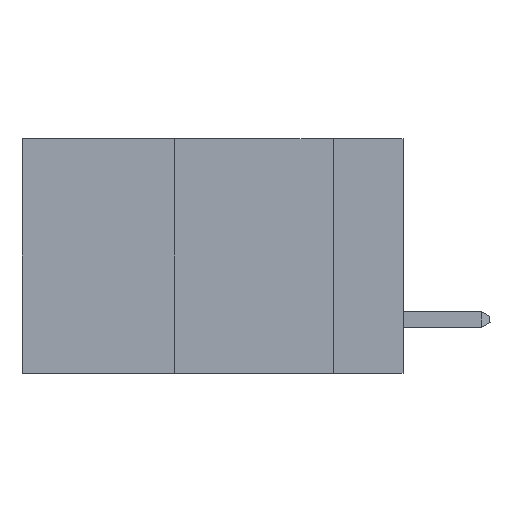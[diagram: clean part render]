
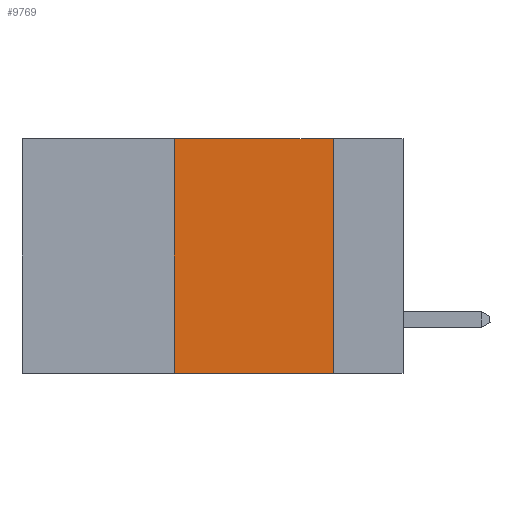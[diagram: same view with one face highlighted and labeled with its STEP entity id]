
A CAD part, left-side view. The second image highlights one B-rep face of the part: STEP entity #9769.
In plain terms, the highlighted planar face has unit normal (-1, 0, 0).
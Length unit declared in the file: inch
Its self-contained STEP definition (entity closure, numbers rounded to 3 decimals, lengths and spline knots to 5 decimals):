
#14 = LINE ( 'NONE', #6779, #7259 ) ;
#136 = VERTEX_POINT ( 'NONE', #248 ) ;
#248 = CARTESIAN_POINT ( 'NONE',  ( 0., 0.11, 0. ) ) ;
#897 = EDGE_CURVE ( 'NONE', #6938, #2614, #8886, .T. ) ;
#1291 = DIRECTION ( 'NONE',  ( 0., 0., -1. ) ) ;
#1312 = ORIENTED_EDGE ( 'NONE', *, *, #897, .F. ) ;
#1478 = VECTOR ( 'NONE', #5497, 39.37008 ) ;
#1621 = VECTOR ( 'NONE', #9694, 39.37008 ) ;
#2044 = DIRECTION ( 'NONE',  ( 0., -1., 0. ) ) ;
#2462 = CARTESIAN_POINT ( 'NONE',  ( 0., 0.11, 0. ) ) ;
#2614 = VERTEX_POINT ( 'NONE', #3173 ) ;
#3173 = CARTESIAN_POINT ( 'NONE',  ( 0., 0.36, 0. ) ) ;
#3242 = EDGE_CURVE ( 'NONE', #2614, #136, #3468, .T. ) ;
#3468 = LINE ( 'NONE', #7407, #1621 ) ;
#3653 = DIRECTION ( 'NONE',  ( 1., 0., 0. ) ) ;
#3674 = CARTESIAN_POINT ( 'NONE',  ( 0., 0.11, -0.37 ) ) ;
#3893 = VECTOR ( 'NONE', #5516, 39.37008 ) ;
#4105 = EDGE_CURVE ( 'NONE', #136, #5055, #6403, .T. ) ;
#4656 = ORIENTED_EDGE ( 'NONE', *, *, #4105, .F. ) ;
#5055 = VERTEX_POINT ( 'NONE', #3674 ) ;
#5153 = CARTESIAN_POINT ( 'NONE',  ( 0., 0.6, 0. ) ) ;
#5247 = PLANE ( 'NONE',  #9955 ) ;
#5497 = DIRECTION ( 'NONE',  ( 0., 0., -1. ) ) ;
#5516 = DIRECTION ( 'NONE',  ( 0., 0., 1. ) ) ;
#5523 = ORIENTED_EDGE ( 'NONE', *, *, #3242, .F. ) ;
#6180 = ORIENTED_EDGE ( 'NONE', *, *, #9826, .T. ) ;
#6403 = LINE ( 'NONE', #2462, #1478 ) ;
#6779 = CARTESIAN_POINT ( 'NONE',  ( 0., 0.6, -0.37 ) ) ;
#6938 = VERTEX_POINT ( 'NONE', #8525 ) ;
#7077 = EDGE_LOOP ( 'NONE', ( #4656, #5523, #1312, #6180 ) ) ;
#7259 = VECTOR ( 'NONE', #2044, 39.37008 ) ;
#7407 = CARTESIAN_POINT ( 'NONE',  ( 0., 0.6, 0. ) ) ;
#8356 = FACE_OUTER_BOUND ( 'NONE', #7077, .T. ) ;
#8525 = CARTESIAN_POINT ( 'NONE',  ( 0., 0.36, -0.37 ) ) ;
#8886 = LINE ( 'NONE', #9247, #3893 ) ;
#9247 = CARTESIAN_POINT ( 'NONE',  ( 0., 0.36, 0. ) ) ;
#9694 = DIRECTION ( 'NONE',  ( 0., -1., 0. ) ) ;
#9769 = ADVANCED_FACE ( 'NONE', ( #8356 ), #5247, .F. ) ;
#9826 = EDGE_CURVE ( 'NONE', #6938, #5055, #14, .T. ) ;
#9955 = AXIS2_PLACEMENT_3D ( 'NONE', #5153, #3653, #1291 ) ;
